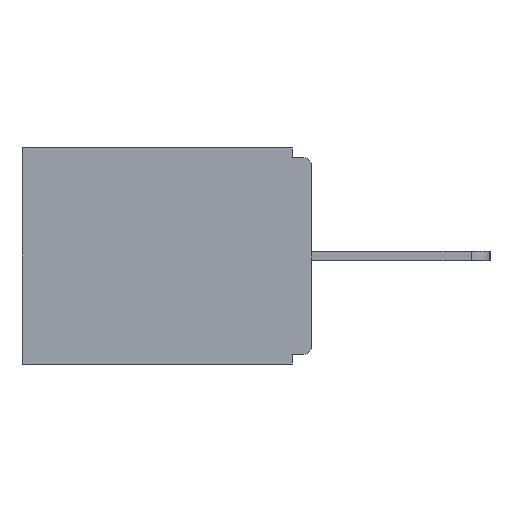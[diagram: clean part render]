
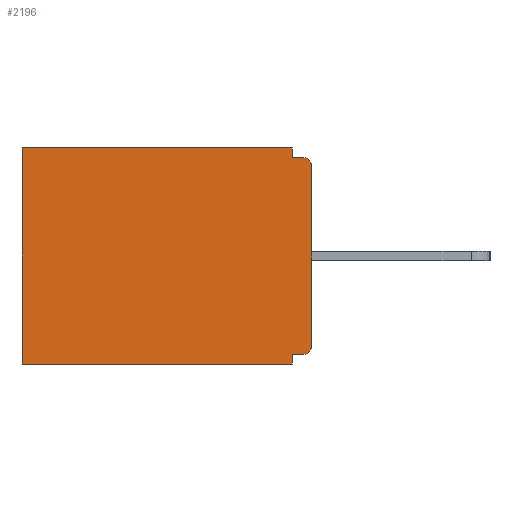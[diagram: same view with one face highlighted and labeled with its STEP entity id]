
A CAD part, left-side view. The second image highlights one B-rep face of the part: STEP entity #2196.
In plain terms, the highlighted planar face has unit normal (-1, 0, 0).
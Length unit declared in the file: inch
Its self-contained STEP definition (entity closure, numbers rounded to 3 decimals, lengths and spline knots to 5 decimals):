
#78 = ORIENTED_EDGE ( 'NONE', *, *, #7181, .T. ) ;
#99 = DIRECTION ( 'NONE',  ( 0., 0., -1. ) ) ;
#265 = LINE ( 'NONE', #6574, #3191 ) ;
#297 = DIRECTION ( 'NONE',  ( 0., 0., -1. ) ) ;
#371 = LINE ( 'NONE', #10624, #2814 ) ;
#717 = CIRCLE ( 'NONE', #9359, 0.015 ) ;
#911 = DIRECTION ( 'NONE',  ( -1., 0., 0. ) ) ;
#1084 = CARTESIAN_POINT ( 'NONE',  ( 0.298, 0.46, 0. ) ) ;
#1343 = VERTEX_POINT ( 'NONE', #7443 ) ;
#1486 = CARTESIAN_POINT ( 'NONE',  ( 0.298, 0., 0. ) ) ;
#1849 = LINE ( 'NONE', #8158, #5312 ) ;
#1914 = DIRECTION ( 'NONE',  ( 0., 1., 0. ) ) ;
#2060 = EDGE_CURVE ( 'NONE', #3376, #13198, #4025, .T. ) ;
#2120 = LINE ( 'NONE', #8372, #11371 ) ;
#2196 = ADVANCED_FACE ( 'NONE', ( #9610 ), #6542, .F. ) ;
#2213 = CARTESIAN_POINT ( 'NONE',  ( 0.298, 0.015, -0.328 ) ) ;
#2384 = DIRECTION ( 'NONE',  ( -1., 0., 0. ) ) ;
#2525 = CARTESIAN_POINT ( 'NONE',  ( 0.298, 0.015, -0.313 ) ) ;
#2814 = VECTOR ( 'NONE', #7416, 39.37008 ) ;
#2852 = VECTOR ( 'NONE', #99, 39.37008 ) ;
#3168 = DIRECTION ( 'NONE',  ( 0., 0., -1. ) ) ;
#3191 = VECTOR ( 'NONE', #4375, 39.37008 ) ;
#3376 = VERTEX_POINT ( 'NONE', #10631 ) ;
#3668 = EDGE_CURVE ( 'NONE', #7655, #10711, #11840, .T. ) ;
#4025 = LINE ( 'NONE', #9352, #6058 ) ;
#4375 = DIRECTION ( 'NONE',  ( 0., -1., 0. ) ) ;
#4438 = ORIENTED_EDGE ( 'NONE', *, *, #9895, .F. ) ;
#4483 = EDGE_CURVE ( 'NONE', #12673, #7551, #7767, .T. ) ;
#5312 = VECTOR ( 'NONE', #6011, 39.37008 ) ;
#5477 = CARTESIAN_POINT ( 'NONE',  ( 0.298, 0.46, -0.343 ) ) ;
#5535 = DIRECTION ( 'NONE',  ( 0., 0., -1. ) ) ;
#5613 = EDGE_CURVE ( 'NONE', #10711, #13276, #8317, .T. ) ;
#5796 = EDGE_CURVE ( 'NONE', #1343, #6839, #265, .T. ) ;
#5931 = CARTESIAN_POINT ( 'NONE',  ( 0.298, 0., -0.03 ) ) ;
#5944 = VECTOR ( 'NONE', #3168, 39.37008 ) ;
#5993 = ORIENTED_EDGE ( 'NONE', *, *, #12255, .F. ) ;
#6011 = DIRECTION ( 'NONE',  ( 0., 0., -1. ) ) ;
#6058 = VECTOR ( 'NONE', #9284, 39.37008 ) ;
#6256 = ORIENTED_EDGE ( 'NONE', *, *, #2060, .F. ) ;
#6542 = PLANE ( 'NONE',  #6859 ) ;
#6574 = CARTESIAN_POINT ( 'NONE',  ( 0.298, 0., -0.015 ) ) ;
#6839 = VERTEX_POINT ( 'NONE', #8915 ) ;
#6859 = AXIS2_PLACEMENT_3D ( 'NONE', #12804, #12729, #297 ) ;
#7113 = ORIENTED_EDGE ( 'NONE', *, *, #4483, .T. ) ;
#7181 = EDGE_CURVE ( 'NONE', #12122, #6839, #717, .T. ) ;
#7416 = DIRECTION ( 'NONE',  ( 0., 1., 0. ) ) ;
#7443 = CARTESIAN_POINT ( 'NONE',  ( 0.298, 0.031, -0.015 ) ) ;
#7551 = VERTEX_POINT ( 'NONE', #9547 ) ;
#7655 = VERTEX_POINT ( 'NONE', #11078 ) ;
#7767 = CIRCLE ( 'NONE', #9483, 0.015 ) ;
#7806 = VECTOR ( 'NONE', #12667, 39.37008 ) ;
#8158 = CARTESIAN_POINT ( 'NONE',  ( 0.298, 0.031, -0.343 ) ) ;
#8283 = CARTESIAN_POINT ( 'NONE',  ( 0.298, 0., 0. ) ) ;
#8317 = LINE ( 'NONE', #13243, #5944 ) ;
#8372 = CARTESIAN_POINT ( 'NONE',  ( 0.298, 0., -0.343 ) ) ;
#8699 = EDGE_LOOP ( 'NONE', ( #78, #8883, #4438, #11510, #13130, #10023, #6256, #11134, #7113, #5993 ) ) ;
#8883 = ORIENTED_EDGE ( 'NONE', *, *, #5796, .F. ) ;
#8915 = CARTESIAN_POINT ( 'NONE',  ( 0.298, 0.015, -0.015 ) ) ;
#9158 = DIRECTION ( 'NONE',  ( 0., 0., -1. ) ) ;
#9284 = DIRECTION ( 'NONE',  ( 0., 0., -1. ) ) ;
#9307 = CARTESIAN_POINT ( 'NONE',  ( 0.298, 0.031, -0.343 ) ) ;
#9352 = CARTESIAN_POINT ( 'NONE',  ( 0.298, 0.031, -0.343 ) ) ;
#9359 = AXIS2_PLACEMENT_3D ( 'NONE', #13087, #911, #9158 ) ;
#9483 = AXIS2_PLACEMENT_3D ( 'NONE', #2525, #2384, #5535 ) ;
#9547 = CARTESIAN_POINT ( 'NONE',  ( 0.298, 0., -0.313 ) ) ;
#9610 = FACE_OUTER_BOUND ( 'NONE', #8699, .T. ) ;
#9895 = EDGE_CURVE ( 'NONE', #7655, #1343, #1849, .T. ) ;
#10023 = ORIENTED_EDGE ( 'NONE', *, *, #11752, .F. ) ;
#10624 = CARTESIAN_POINT ( 'NONE',  ( 0.298, 0., -0.328 ) ) ;
#10631 = CARTESIAN_POINT ( 'NONE',  ( 0.298, 0.031, -0.328 ) ) ;
#10711 = VERTEX_POINT ( 'NONE', #1084 ) ;
#11078 = CARTESIAN_POINT ( 'NONE',  ( 0.298, 0.031, 0. ) ) ;
#11134 = ORIENTED_EDGE ( 'NONE', *, *, #12442, .F. ) ;
#11371 = VECTOR ( 'NONE', #1914, 39.37008 ) ;
#11510 = ORIENTED_EDGE ( 'NONE', *, *, #3668, .T. ) ;
#11752 = EDGE_CURVE ( 'NONE', #13198, #13276, #2120, .T. ) ;
#11840 = LINE ( 'NONE', #1486, #7806 ) ;
#12122 = VERTEX_POINT ( 'NONE', #5931 ) ;
#12255 = EDGE_CURVE ( 'NONE', #12122, #7551, #12275, .T. ) ;
#12275 = LINE ( 'NONE', #8283, #2852 ) ;
#12442 = EDGE_CURVE ( 'NONE', #12673, #3376, #371, .T. ) ;
#12667 = DIRECTION ( 'NONE',  ( 0., 1., 0. ) ) ;
#12673 = VERTEX_POINT ( 'NONE', #2213 ) ;
#12729 = DIRECTION ( 'NONE',  ( 1., 0., 0. ) ) ;
#12804 = CARTESIAN_POINT ( 'NONE',  ( 0.298, 0., 0. ) ) ;
#13087 = CARTESIAN_POINT ( 'NONE',  ( 0.298, 0.015, -0.03 ) ) ;
#13130 = ORIENTED_EDGE ( 'NONE', *, *, #5613, .T. ) ;
#13198 = VERTEX_POINT ( 'NONE', #9307 ) ;
#13243 = CARTESIAN_POINT ( 'NONE',  ( 0.298, 0.46, 0. ) ) ;
#13276 = VERTEX_POINT ( 'NONE', #5477 ) ;
